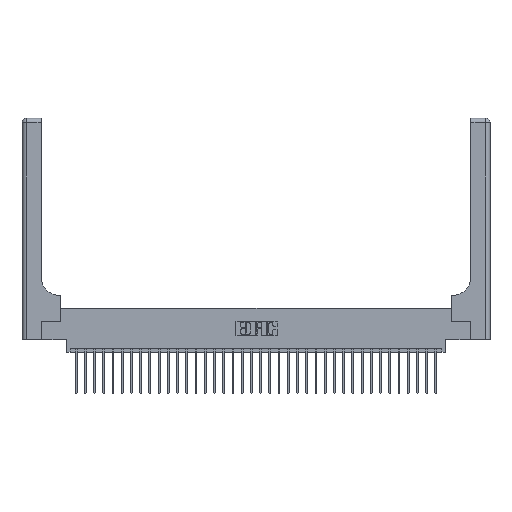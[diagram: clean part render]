
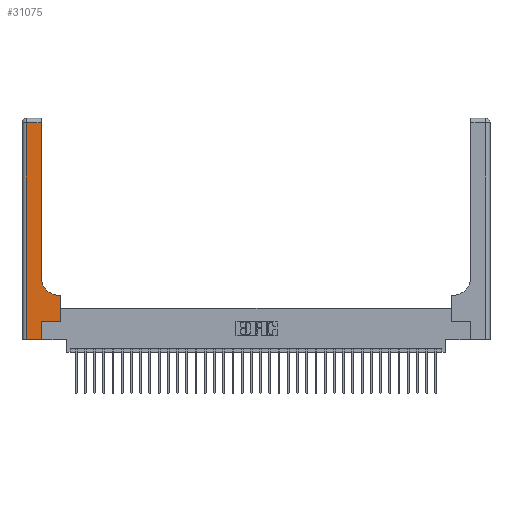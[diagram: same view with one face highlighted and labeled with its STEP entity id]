
A CAD part, top view. The second image highlights one B-rep face of the part: STEP entity #31075.
In plain terms, the highlighted planar face has unit normal (0, 0, 1).
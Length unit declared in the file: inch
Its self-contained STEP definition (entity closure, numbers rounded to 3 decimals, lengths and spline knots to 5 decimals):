
#239 = ORIENTED_EDGE ( 'NONE', *, *, #10798, .T. ) ;
#255 = VERTEX_POINT ( 'NONE', #3109 ) ;
#829 = EDGE_CURVE ( 'NONE', #17403, #20969, #1281, .T. ) ;
#1084 = DIRECTION ( 'NONE',  ( -1., 0., 0. ) ) ;
#1101 = CARTESIAN_POINT ( 'NONE',  ( 0.26, 0.6, 0.37 ) ) ;
#1281 = LINE ( 'NONE', #21462, #8722 ) ;
#2109 = DIRECTION ( 'NONE',  ( 1., 0., 0. ) ) ;
#2131 = CARTESIAN_POINT ( 'NONE',  ( 0.26, 3., 0.37 ) ) ;
#2171 = AXIS2_PLACEMENT_3D ( 'NONE', #4401, #11876, #2109 ) ;
#2189 = CARTESIAN_POINT ( 'NONE',  ( 0.528, 0.25, 0.37 ) ) ;
#2302 = ORIENTED_EDGE ( 'NONE', *, *, #829, .T. ) ;
#3109 = CARTESIAN_POINT ( 'NONE',  ( 0.26, 2.94, 0.37 ) ) ;
#3383 = PLANE ( 'NONE',  #31224 ) ;
#3534 = LINE ( 'NONE', #1101, #13970 ) ;
#4401 = CARTESIAN_POINT ( 'NONE',  ( 0.51, 0.85, 0.37 ) ) ;
#4441 = VECTOR ( 'NONE', #13214, 39.37008 ) ;
#5191 = CARTESIAN_POINT ( 'NONE',  ( 0., 2.94, 0.37 ) ) ;
#6070 = CARTESIAN_POINT ( 'NONE',  ( 0.265, 0.25, 0.37 ) ) ;
#6491 = EDGE_CURVE ( 'NONE', #255, #21590, #31716, .T. ) ;
#6630 = EDGE_CURVE ( 'NONE', #18448, #7355, #3534, .T. ) ;
#7355 = VERTEX_POINT ( 'NONE', #8021 ) ;
#7480 = EDGE_CURVE ( 'NONE', #20969, #10875, #31424, .T. ) ;
#8021 = CARTESIAN_POINT ( 'NONE',  ( 0.51, 0.6, 0.37 ) ) ;
#8722 = VECTOR ( 'NONE', #31210, 39.37008 ) ;
#8993 = CARTESIAN_POINT ( 'NONE',  ( 0.265, 0., 0.37 ) ) ;
#9153 = DIRECTION ( 'NONE',  ( 0., 1., 0. ) ) ;
#9384 = VECTOR ( 'NONE', #9153, 39.37008 ) ;
#9622 = DIRECTION ( 'NONE',  ( -1., 0., 0. ) ) ;
#10798 = EDGE_CURVE ( 'NONE', #21590, #17403, #15150, .T. ) ;
#10875 = VERTEX_POINT ( 'NONE', #12574 ) ;
#10877 = DIRECTION ( 'NONE',  ( 0., 0., -1. ) ) ;
#11352 = ORIENTED_EDGE ( 'NONE', *, *, #18391, .T. ) ;
#11809 = DIRECTION ( 'NONE',  ( -1., 0., 0. ) ) ;
#11876 = DIRECTION ( 'NONE',  ( 0., 0., -1. ) ) ;
#12574 = CARTESIAN_POINT ( 'NONE',  ( 0.265, 0.25, 0.37 ) ) ;
#13214 = DIRECTION ( 'NONE',  ( 0., -1., 0. ) ) ;
#13970 = VECTOR ( 'NONE', #11809, 39.37008 ) ;
#14514 = LINE ( 'NONE', #22176, #26858 ) ;
#14885 = ORIENTED_EDGE ( 'NONE', *, *, #29106, .T. ) ;
#15150 = LINE ( 'NONE', #27682, #4441 ) ;
#15967 = DIRECTION ( 'NONE',  ( 1., 0., 0. ) ) ;
#16039 = CARTESIAN_POINT ( 'NONE',  ( 0., 3., 0.37 ) ) ;
#16515 = FACE_OUTER_BOUND ( 'NONE', #22065, .T. ) ;
#16621 = CARTESIAN_POINT ( 'NONE',  ( 0.06, 0., 0.37 ) ) ;
#17102 = VECTOR ( 'NONE', #15967, 39.37008 ) ;
#17114 = DIRECTION ( 'NONE',  ( 0., 1., 0. ) ) ;
#17403 = VERTEX_POINT ( 'NONE', #16621 ) ;
#17568 = CARTESIAN_POINT ( 'NONE',  ( 0.06, 2.94, 0.37 ) ) ;
#18391 = EDGE_CURVE ( 'NONE', #19727, #18448, #14514, .T. ) ;
#18448 = VERTEX_POINT ( 'NONE', #29969 ) ;
#18769 = EDGE_CURVE ( 'NONE', #10875, #19727, #28351, .T. ) ;
#19038 = ORIENTED_EDGE ( 'NONE', *, *, #20646, .T. ) ;
#19727 = VERTEX_POINT ( 'NONE', #2189 ) ;
#20646 = EDGE_CURVE ( 'NONE', #7355, #24005, #26063, .T. ) ;
#20969 = VERTEX_POINT ( 'NONE', #21118 ) ;
#21118 = CARTESIAN_POINT ( 'NONE',  ( 0.265, 0., 0.37 ) ) ;
#21462 = CARTESIAN_POINT ( 'NONE',  ( 0., 0., 0.37 ) ) ;
#21586 = ORIENTED_EDGE ( 'NONE', *, *, #18769, .T. ) ;
#21590 = VERTEX_POINT ( 'NONE', #17568 ) ;
#22065 = EDGE_LOOP ( 'NONE', ( #14885, #23414, #239, #2302, #26114, #21586, #11352, #31092, #19038 ) ) ;
#22176 = CARTESIAN_POINT ( 'NONE',  ( 0.528, 0.25, 0.37 ) ) ;
#23358 = CARTESIAN_POINT ( 'NONE',  ( 0.26, 0.85, 0.37 ) ) ;
#23414 = ORIENTED_EDGE ( 'NONE', *, *, #6491, .T. ) ;
#24005 = VERTEX_POINT ( 'NONE', #23358 ) ;
#26063 = CIRCLE ( 'NONE', #2171, 0.25 ) ;
#26114 = ORIENTED_EDGE ( 'NONE', *, *, #7480, .T. ) ;
#26701 = LINE ( 'NONE', #2131, #28617 ) ;
#26858 = VECTOR ( 'NONE', #17114, 39.37008 ) ;
#27333 = DIRECTION ( 'NONE',  ( 0., 1., 0. ) ) ;
#27682 = CARTESIAN_POINT ( 'NONE',  ( 0.06, 3., 0.37 ) ) ;
#27999 = VECTOR ( 'NONE', #9622, 39.37008 ) ;
#28351 = LINE ( 'NONE', #6070, #17102 ) ;
#28617 = VECTOR ( 'NONE', #27333, 39.37008 ) ;
#29106 = EDGE_CURVE ( 'NONE', #24005, #255, #26701, .T. ) ;
#29969 = CARTESIAN_POINT ( 'NONE',  ( 0.528, 0.6, 0.37 ) ) ;
#31075 = ADVANCED_FACE ( 'NONE', ( #16515 ), #3383, .F. ) ;
#31092 = ORIENTED_EDGE ( 'NONE', *, *, #6630, .T. ) ;
#31210 = DIRECTION ( 'NONE',  ( 1., 0., 0. ) ) ;
#31224 = AXIS2_PLACEMENT_3D ( 'NONE', #16039, #10877, #1084 ) ;
#31424 = LINE ( 'NONE', #8993, #9384 ) ;
#31716 = LINE ( 'NONE', #5191, #27999 ) ;
